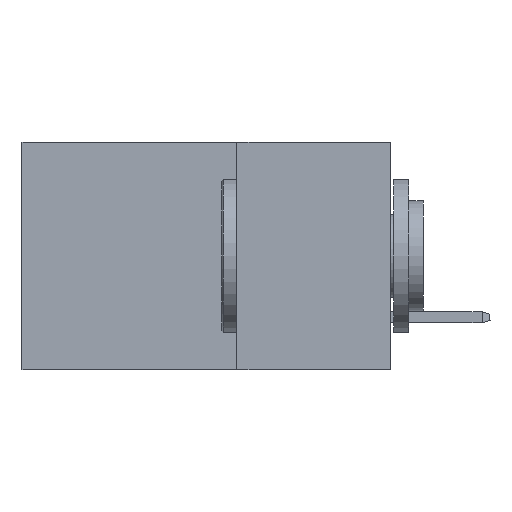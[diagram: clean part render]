
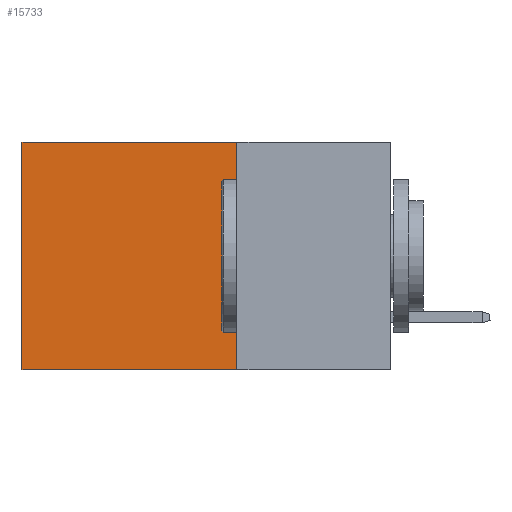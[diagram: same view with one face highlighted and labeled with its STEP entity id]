
A CAD part, left-side view. The second image highlights one B-rep face of the part: STEP entity #15733.
In plain terms, the highlighted planar face has unit normal (-1, 0, 0).
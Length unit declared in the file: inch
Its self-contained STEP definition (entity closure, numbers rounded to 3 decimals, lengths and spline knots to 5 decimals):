
#1059 = ORIENTED_EDGE ( 'NONE', *, *, #26423, .F. ) ;
#1414 = FACE_OUTER_BOUND ( 'NONE', #17503, .T. ) ;
#1487 = DIRECTION ( 'NONE',  ( 0., 0., -1. ) ) ;
#2208 = LINE ( 'NONE', #24491, #26434 ) ;
#2906 = DIRECTION ( 'NONE',  ( 1., 0., 0. ) ) ;
#3117 = CARTESIAN_POINT ( 'NONE',  ( 0.2875, 0.25, 0. ) ) ;
#5268 = CARTESIAN_POINT ( 'NONE',  ( 0.2875, 0.6, 0. ) ) ;
#5526 = CARTESIAN_POINT ( 'NONE',  ( 0.2875, 0.25, -0.37 ) ) ;
#5651 = CARTESIAN_POINT ( 'NONE',  ( 0.2875, 0.6, -0.37 ) ) ;
#9206 = AXIS2_PLACEMENT_3D ( 'NONE', #3117, #2906, #28771 ) ;
#9365 = VECTOR ( 'NONE', #1487, 39.37008 ) ;
#11268 = VECTOR ( 'NONE', #19506, 39.37008 ) ;
#11773 = DIRECTION ( 'NONE',  ( 0., 1., 0. ) ) ;
#11864 = ORIENTED_EDGE ( 'NONE', *, *, #13910, .T. ) ;
#12056 = CARTESIAN_POINT ( 'NONE',  ( 0.2875, 0.25, 0. ) ) ;
#12199 = CARTESIAN_POINT ( 'NONE',  ( 0.2875, 0.25, 0. ) ) ;
#13602 = VERTEX_POINT ( 'NONE', #5526 ) ;
#13910 = EDGE_CURVE ( 'NONE', #29883, #24370, #21197, .T. ) ;
#15733 = ADVANCED_FACE ( 'NONE', ( #1414 ), #30048, .F. ) ;
#17139 = VECTOR ( 'NONE', #11773, 39.37008 ) ;
#17382 = EDGE_CURVE ( 'NONE', #24370, #20947, #28879, .T. ) ;
#17503 = EDGE_LOOP ( 'NONE', ( #28644, #1059, #24154, #11864 ) ) ;
#17798 = LINE ( 'NONE', #12056, #9365 ) ;
#18142 = EDGE_CURVE ( 'NONE', #29883, #13602, #17798, .T. ) ;
#19506 = DIRECTION ( 'NONE',  ( 0., 0., -1. ) ) ;
#20947 = VERTEX_POINT ( 'NONE', #5651 ) ;
#21095 = CARTESIAN_POINT ( 'NONE',  ( 0.2875, 0.25, 0. ) ) ;
#21197 = LINE ( 'NONE', #21095, #17139 ) ;
#24154 = ORIENTED_EDGE ( 'NONE', *, *, #18142, .F. ) ;
#24370 = VERTEX_POINT ( 'NONE', #29433 ) ;
#24491 = CARTESIAN_POINT ( 'NONE',  ( 0.2875, 0.25, -0.37 ) ) ;
#26423 = EDGE_CURVE ( 'NONE', #13602, #20947, #2208, .T. ) ;
#26434 = VECTOR ( 'NONE', #27264, 39.37008 ) ;
#27264 = DIRECTION ( 'NONE',  ( 0., 1., 0. ) ) ;
#28644 = ORIENTED_EDGE ( 'NONE', *, *, #17382, .T. ) ;
#28771 = DIRECTION ( 'NONE',  ( 0., 0., -1. ) ) ;
#28879 = LINE ( 'NONE', #5268, #11268 ) ;
#29433 = CARTESIAN_POINT ( 'NONE',  ( 0.2875, 0.6, 0. ) ) ;
#29883 = VERTEX_POINT ( 'NONE', #12199 ) ;
#30048 = PLANE ( 'NONE',  #9206 ) ;
